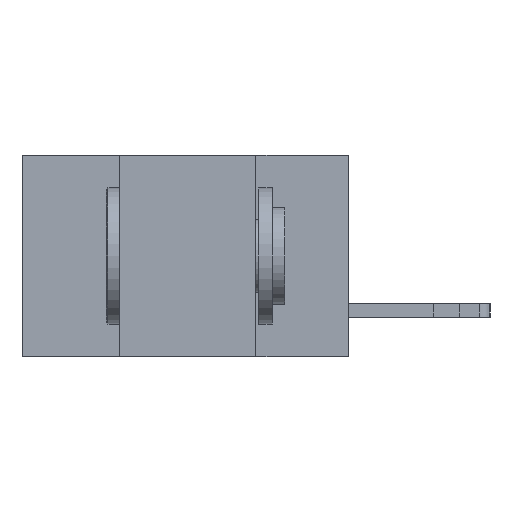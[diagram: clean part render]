
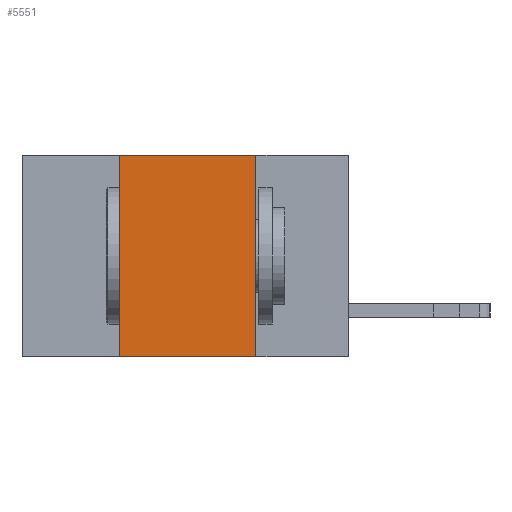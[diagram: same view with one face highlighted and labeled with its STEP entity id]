
A CAD part, left-side view. The second image highlights one B-rep face of the part: STEP entity #5551.
In plain terms, the highlighted planar face has unit normal (-1, 0, 0).
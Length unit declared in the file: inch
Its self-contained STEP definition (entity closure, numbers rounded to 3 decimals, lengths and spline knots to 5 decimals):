
#452 = DIRECTION ( 'NONE',  ( 0., 0., 1. ) ) ;
#847 = EDGE_CURVE ( 'NONE', #11551, #2175, #2166, .T. ) ;
#991 = VECTOR ( 'NONE', #3073, 39.37008 ) ;
#1627 = CARTESIAN_POINT ( 'NONE',  ( 0., 0.17, -0.37 ) ) ;
#1695 = DIRECTION ( 'NONE',  ( 0., 0., -1. ) ) ;
#1862 = AXIS2_PLACEMENT_3D ( 'NONE', #2762, #4007, #1695 ) ;
#2056 = EDGE_CURVE ( 'NONE', #4016, #11551, #6629, .T. ) ;
#2166 = LINE ( 'NONE', #5272, #12977 ) ;
#2175 = VERTEX_POINT ( 'NONE', #1627 ) ;
#2241 = CARTESIAN_POINT ( 'NONE',  ( 0., 0.6, -0.37 ) ) ;
#2556 = ORIENTED_EDGE ( 'NONE', *, *, #2056, .F. ) ;
#2762 = CARTESIAN_POINT ( 'NONE',  ( 0., 0.6, 0. ) ) ;
#3027 = CARTESIAN_POINT ( 'NONE',  ( 0., 0.42, -0.37 ) ) ;
#3073 = DIRECTION ( 'NONE',  ( 0., -1., 0. ) ) ;
#3237 = CARTESIAN_POINT ( 'NONE',  ( 0., 0.42, 0. ) ) ;
#4007 = DIRECTION ( 'NONE',  ( 1., 0., 0. ) ) ;
#4016 = VERTEX_POINT ( 'NONE', #3237 ) ;
#4351 = ORIENTED_EDGE ( 'NONE', *, *, #847, .F. ) ;
#4516 = ORIENTED_EDGE ( 'NONE', *, *, #12366, .F. ) ;
#5272 = CARTESIAN_POINT ( 'NONE',  ( 0., 0.17, 0. ) ) ;
#5341 = LINE ( 'NONE', #6798, #8218 ) ;
#5551 = ADVANCED_FACE ( 'NONE', ( #11334 ), #11468, .F. ) ;
#6254 = VECTOR ( 'NONE', #7559, 39.37008 ) ;
#6587 = LINE ( 'NONE', #2241, #6254 ) ;
#6629 = LINE ( 'NONE', #10119, #991 ) ;
#6798 = CARTESIAN_POINT ( 'NONE',  ( 0., 0.42, 0. ) ) ;
#7559 = DIRECTION ( 'NONE',  ( 0., -1., 0. ) ) ;
#8218 = VECTOR ( 'NONE', #452, 39.37008 ) ;
#9030 = VERTEX_POINT ( 'NONE', #3027 ) ;
#9168 = EDGE_LOOP ( 'NONE', ( #4351, #2556, #4516, #11378 ) ) ;
#9467 = DIRECTION ( 'NONE',  ( 0., 0., -1. ) ) ;
#10119 = CARTESIAN_POINT ( 'NONE',  ( 0., 0.6, 0. ) ) ;
#11334 = FACE_OUTER_BOUND ( 'NONE', #9168, .T. ) ;
#11378 = ORIENTED_EDGE ( 'NONE', *, *, #11686, .T. ) ;
#11468 = PLANE ( 'NONE',  #1862 ) ;
#11551 = VERTEX_POINT ( 'NONE', #12442 ) ;
#11686 = EDGE_CURVE ( 'NONE', #9030, #2175, #6587, .T. ) ;
#12366 = EDGE_CURVE ( 'NONE', #9030, #4016, #5341, .T. ) ;
#12442 = CARTESIAN_POINT ( 'NONE',  ( 0., 0.17, 0. ) ) ;
#12977 = VECTOR ( 'NONE', #9467, 39.37008 ) ;
